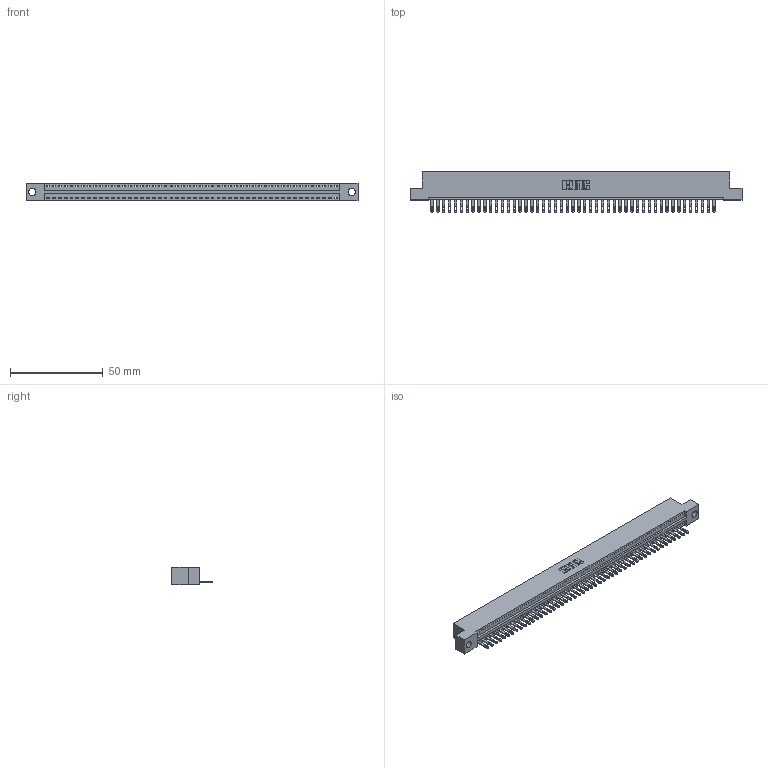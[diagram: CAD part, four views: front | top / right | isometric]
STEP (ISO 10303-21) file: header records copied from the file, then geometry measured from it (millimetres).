
FILE_DESCRIPTION (( 'STEP AP203' ), '1' );
FILE_NAME ('896-050-500-104.STEP', '2021-07-27T23:25:04', ( '' ), ( '' ), 'SwSTEP 2.0', 'SolidWorks 2020', '' );
FILE_SCHEMA (( 'CONFIG_CONTROL_DESIGN' ));
Length unit declared in the file: inch
Products named in the file (3): 896-050-500-104; 846 Part_Flush Mounting Lugs - 0.156 Dia-TH; 345-292-001_345-293-100
Assembly tree (50 placements, depth 2):
  896-050-500-104
    846 Part_Flush Mounting Lugs - 0.156 Dia-TH
    345-292-001_345-293-100  x49
Bounding box: 179.32 x 21.84 x 9.4 mm (x, y, z)
Volume: 17151.4 mm3; surface area: 21381 mm2
Topology: 50 solids, 50 shells, 2780 faces, 8603 edges, 5734 vertices
Faces by surface type: plane 1752, cylinder 1028
Entity records: 29855 total; most frequent: CARTESIAN_POINT 5125, ORIENTED_EDGE 5110, DIRECTION 4513, EDGE_CURVE 2555, VECTOR 2219, LINE 2219, VERTEX_POINT 1702, AXIS2_PLACEMENT_3D 1147
